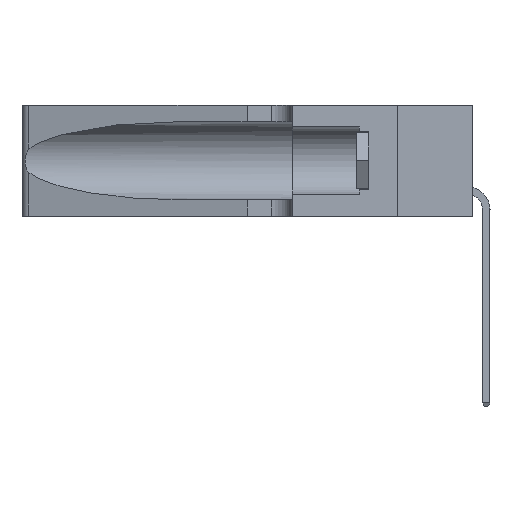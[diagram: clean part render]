
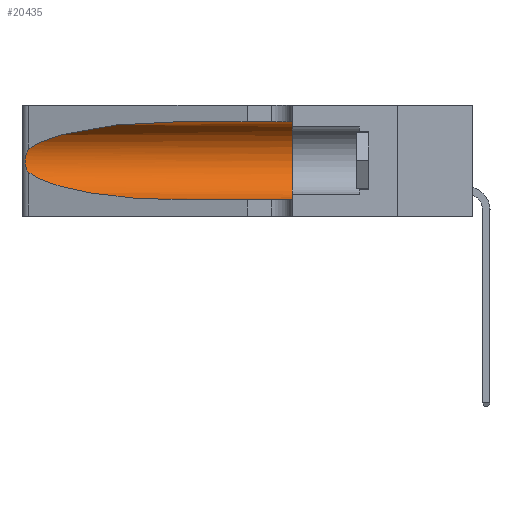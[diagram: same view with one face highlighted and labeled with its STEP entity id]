
A CAD part, left-side view. The second image highlights one B-rep face of the part: STEP entity #20435.
In plain terms, the highlighted cylindrical face has radius 3.308 mm (diameter 6.617 mm), a partial arc.
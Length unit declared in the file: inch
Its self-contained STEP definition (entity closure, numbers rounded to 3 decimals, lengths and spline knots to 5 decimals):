
#352 = CARTESIAN_POINT ( 'NONE',  ( 0.25789, 1.23486, 0.15765 ) ) ;
#2000 = CARTESIAN_POINT ( 'NONE',  ( 0.1305, 1.61858, 0.05475 ) ) ;
#2015 = DIRECTION ( 'NONE',  ( 0., -1., 0. ) ) ;
#3216 = CARTESIAN_POINT ( 'NONE',  ( 0.18966, 0.96281, 0.05475 ) ) ;
#3479 = CARTESIAN_POINT ( 'NONE',  ( 0.2373, 1.15595, 0.28018 ) ) ;
#3759 = ORIENTED_EDGE ( 'NONE', *, *, #18049, .T. ) ;
#4757 = CARTESIAN_POINT ( 'NONE',  ( 0.1305, 0.35, 0.31525 ) ) ;
#5335 = DIRECTION ( 'NONE',  ( 0., -1., 0. ) ) ;
#5351 =( BOUNDED_CURVE ( )  B_SPLINE_CURVE ( 3, ( #23288, #33271, #3216, #6509 ),
 .UNSPECIFIED., .F., .T. ) 
 B_SPLINE_CURVE_WITH_KNOTS ( ( 4, 4 ),
 ( 3.44316, 4.71239 ),
 .UNSPECIFIED. ) 
 CURVE ( )  GEOMETRIC_REPRESENTATION_ITEM ( )  RATIONAL_B_SPLINE_CURVE ( ( 1., 0.87, 0.87, 1. ) ) 
 REPRESENTATION_ITEM ( '' )  );
#5733 = CARTESIAN_POINT ( 'NONE',  ( 0.1305, 0.72297, 0.31525 ) ) ;
#6164 = CARTESIAN_POINT ( 'NONE',  ( 0.25639, 1.23184, 0.21858 ) ) ;
#6509 = CARTESIAN_POINT ( 'NONE',  ( 0.1305, 0.72297, 0.05475 ) ) ;
#6675 = CARTESIAN_POINT ( 'NONE',  ( 0.25555, 1.22993, 0.14849 ) ) ;
#6804 = CARTESIAN_POINT ( 'NONE',  ( 0.25487, 1.22718, 0.14631 ) ) ;
#7061 = CARTESIAN_POINT ( 'NONE',  ( 0.1305, 0.72297, 0.31525 ) ) ;
#7086 = CARTESIAN_POINT ( 'NONE',  ( 0.25639, 1.23186, 0.15144 ) ) ;
#8503 = AXIS2_PLACEMENT_3D ( 'NONE', #21790, #25107, #18733 ) ;
#8702 = CARTESIAN_POINT ( 'NONE',  ( 0.1305, 0.72297, 0.05475 ) ) ;
#8741 = DIRECTION ( 'NONE',  ( 0., -1., 0. ) ) ;
#8905 = FACE_OUTER_BOUND ( 'NONE', #36032, .T. ) ;
#9931 = VERTEX_POINT ( 'NONE', #18243 ) ;
#9942 = VERTEX_POINT ( 'NONE', #15187 ) ;
#11546 = VERTEX_POINT ( 'NONE', #8702 ) ;
#12318 = VECTOR ( 'NONE', #8741, 39.37008 ) ;
#12661 = CIRCLE ( 'NONE', #8503, 0.13025 ) ;
#13256 = LINE ( 'NONE', #2000, #16410 ) ;
#13943 =( BOUNDED_CURVE ( )  B_SPLINE_CURVE ( 3, ( #5733, #28795, #3479, #33041 ),
 .UNSPECIFIED., .F., .T. ) 
 B_SPLINE_CURVE_WITH_KNOTS ( ( 4, 4 ),
 ( 1.5708, 2.84003 ),
 .UNSPECIFIED. ) 
 CURVE ( )  GEOMETRIC_REPRESENTATION_ITEM ( )  RATIONAL_B_SPLINE_CURVE ( ( 1., 0.87, 0.87, 1. ) ) 
 REPRESENTATION_ITEM ( '' )  );
#15187 = CARTESIAN_POINT ( 'NONE',  ( 0.1305, 0.35, 0.05475 ) ) ;
#16112 = CARTESIAN_POINT ( 'NONE',  ( 0.26018, 1.23835, 0.19895 ) ) ;
#16410 = VECTOR ( 'NONE', #5335, 39.37008 ) ;
#18049 = EDGE_CURVE ( 'NONE', #39213, #11546, #5351, .T. ) ;
#18243 = CARTESIAN_POINT ( 'NONE',  ( 0.25487, 1.22718, 0.22369 ) ) ;
#18364 = VERTEX_POINT ( 'NONE', #4757 ) ;
#18733 = DIRECTION ( 'NONE',  ( 0., 0., 1. ) ) ;
#19293 = CARTESIAN_POINT ( 'NONE',  ( 0.25555, 1.22994, 0.2215 ) ) ;
#19702 = CARTESIAN_POINT ( 'NONE',  ( 0.25787, 1.23484, 0.2124 ) ) ;
#20435 = ADVANCED_FACE ( 'NONE', ( #8905 ), #20766, .F. ) ;
#20766 = CYLINDRICAL_SURFACE ( 'NONE', #40470, 0.13025 ) ;
#21790 = CARTESIAN_POINT ( 'NONE',  ( 0.1305, 0.35, 0.185 ) ) ;
#21820 = CARTESIAN_POINT ( 'NONE',  ( 0.1305, 1.61858, 0.185 ) ) ;
#22811 = EDGE_CURVE ( 'NONE', #25678, #18364, #28383, .T. ) ;
#23288 = CARTESIAN_POINT ( 'NONE',  ( 0.25487, 1.22718, 0.14631 ) ) ;
#25107 = DIRECTION ( 'NONE',  ( 0., 1., 0. ) ) ;
#25678 = VERTEX_POINT ( 'NONE', #7061 ) ;
#28383 = LINE ( 'NONE', #34943, #12318 ) ;
#28795 = CARTESIAN_POINT ( 'NONE',  ( 0.18966, 0.96281, 0.31525 ) ) ;
#29698 = EDGE_CURVE ( 'NONE', #18364, #9942, #12661, .T. ) ;
#31337 = EDGE_CURVE ( 'NONE', #11546, #9942, #13256, .T. ) ;
#31478 = EDGE_CURVE ( 'NONE', #9931, #39213, #37168, .T. ) ;
#32076 = ORIENTED_EDGE ( 'NONE', *, *, #40586, .T. ) ;
#32668 = DIRECTION ( 'NONE',  ( 0., 0., -1. ) ) ;
#33041 = CARTESIAN_POINT ( 'NONE',  ( 0.25487, 1.22718, 0.22369 ) ) ;
#33271 = CARTESIAN_POINT ( 'NONE',  ( 0.2373, 1.15595, 0.08982 ) ) ;
#34943 = CARTESIAN_POINT ( 'NONE',  ( 0.1305, 1.61858, 0.31525 ) ) ;
#35792 = CARTESIAN_POINT ( 'NONE',  ( 0.25854, 1.2359, 0.20912 ) ) ;
#35882 = ORIENTED_EDGE ( 'NONE', *, *, #31337, .T. ) ;
#36032 = EDGE_LOOP ( 'NONE', ( #32076, #37539, #3759, #35882, #38353, #41691 ) ) ;
#37168 = B_SPLINE_CURVE_WITH_KNOTS ( 'NONE', 3,
 ( #38948, #19293, #6164, #19702, #35792, #16112, #42339, #39219, #42475, #39991, #352, #7086, #6675, #6804 ),
 .UNSPECIFIED., .F., .F.,
 ( 4, 2, 2, 2, 2, 2, 4 ),
 ( 0., 0.00027, 0.00053, 0.00107, 0.0016, 0.00187, 0.00214 ),
 .UNSPECIFIED. ) ;
#37539 = ORIENTED_EDGE ( 'NONE', *, *, #31478, .T. ) ;
#38238 = CARTESIAN_POINT ( 'NONE',  ( 0.25487, 1.22718, 0.14631 ) ) ;
#38353 = ORIENTED_EDGE ( 'NONE', *, *, #29698, .F. ) ;
#38948 = CARTESIAN_POINT ( 'NONE',  ( 0.25487, 1.22718, 0.22369 ) ) ;
#39213 = VERTEX_POINT ( 'NONE', #38238 ) ;
#39219 = CARTESIAN_POINT ( 'NONE',  ( 0.26075, 1.23896, 0.178 ) ) ;
#39991 = CARTESIAN_POINT ( 'NONE',  ( 0.25856, 1.23593, 0.16098 ) ) ;
#40470 = AXIS2_PLACEMENT_3D ( 'NONE', #21820, #2015, #32668 ) ;
#40586 = EDGE_CURVE ( 'NONE', #25678, #9931, #13943, .T. ) ;
#41691 = ORIENTED_EDGE ( 'NONE', *, *, #22811, .F. ) ;
#42339 = CARTESIAN_POINT ( 'NONE',  ( 0.26075, 1.23896, 0.19203 ) ) ;
#42475 = CARTESIAN_POINT ( 'NONE',  ( 0.26017, 1.23833, 0.17102 ) ) ;
